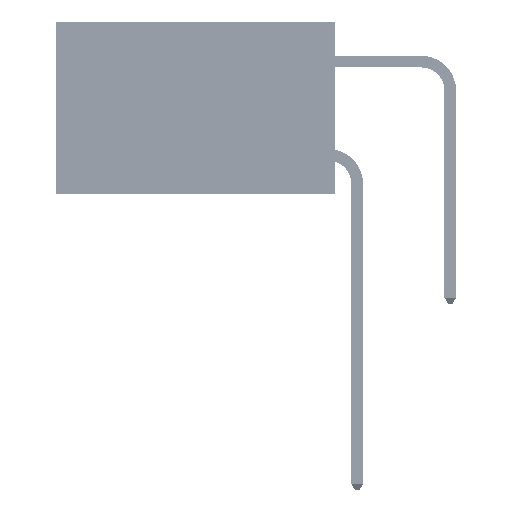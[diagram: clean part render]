
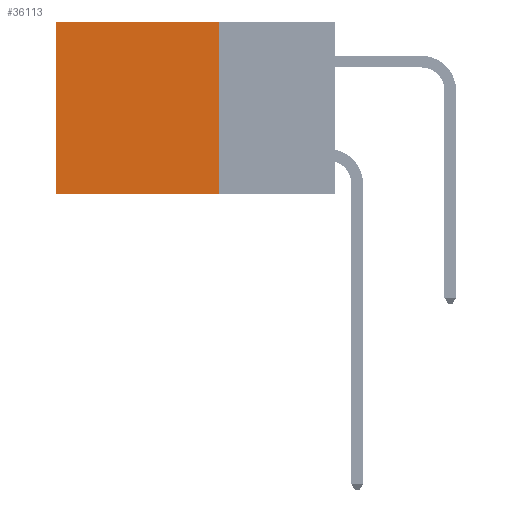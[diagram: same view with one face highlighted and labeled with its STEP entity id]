
A CAD part, left-side view. The second image highlights one B-rep face of the part: STEP entity #36113.
In plain terms, the highlighted planar face has unit normal (-1, 0, 0).
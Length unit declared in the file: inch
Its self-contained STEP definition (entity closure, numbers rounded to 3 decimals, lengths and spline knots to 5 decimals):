
#120 = CARTESIAN_POINT ( 'NONE',  ( 0.2875, 0.25, -0.37 ) ) ;
#1273 = DIRECTION ( 'NONE',  ( 0., 1., 0. ) ) ;
#5257 = EDGE_CURVE ( 'NONE', #51670, #51236, #9615, .T. ) ;
#5672 = DIRECTION ( 'NONE',  ( 1., 0., 0. ) ) ;
#8105 = CARTESIAN_POINT ( 'NONE',  ( 0.2875, 0.25, 0. ) ) ;
#9615 = LINE ( 'NONE', #45702, #12149 ) ;
#9838 = EDGE_LOOP ( 'NONE', ( #26033, #38662, #48596, #29045 ) ) ;
#12149 = VECTOR ( 'NONE', #1273, 39.37008 ) ;
#16026 = EDGE_CURVE ( 'NONE', #17671, #51670, #20615, .T. ) ;
#16264 = EDGE_CURVE ( 'NONE', #17671, #49271, #29444, .T. ) ;
#17465 = VECTOR ( 'NONE', #42611, 39.37008 ) ;
#17671 = VERTEX_POINT ( 'NONE', #19517 ) ;
#19517 = CARTESIAN_POINT ( 'NONE',  ( 0.2875, 0.25, 0. ) ) ;
#20615 = LINE ( 'NONE', #30305, #17465 ) ;
#21214 = CARTESIAN_POINT ( 'NONE',  ( 0.2875, 0.6, -0.37 ) ) ;
#21512 = CARTESIAN_POINT ( 'NONE',  ( 0.2875, 0.25, 0. ) ) ;
#22758 = LINE ( 'NONE', #32452, #39108 ) ;
#25727 = AXIS2_PLACEMENT_3D ( 'NONE', #21512, #5672, #46287 ) ;
#25748 = PLANE ( 'NONE',  #25727 ) ;
#26033 = ORIENTED_EDGE ( 'NONE', *, *, #27079, .T. ) ;
#27079 = EDGE_CURVE ( 'NONE', #49271, #51236, #22758, .T. ) ;
#27839 = DIRECTION ( 'NONE',  ( 0., 1., 0. ) ) ;
#29045 = ORIENTED_EDGE ( 'NONE', *, *, #16264, .T. ) ;
#29444 = LINE ( 'NONE', #8105, #42043 ) ;
#30305 = CARTESIAN_POINT ( 'NONE',  ( 0.2875, 0.25, 0. ) ) ;
#32452 = CARTESIAN_POINT ( 'NONE',  ( 0.2875, 0.6, 0. ) ) ;
#36113 = ADVANCED_FACE ( 'NONE', ( #39462 ), #25748, .F. ) ;
#38662 = ORIENTED_EDGE ( 'NONE', *, *, #5257, .F. ) ;
#39108 = VECTOR ( 'NONE', #48640, 39.37008 ) ;
#39462 = FACE_OUTER_BOUND ( 'NONE', #9838, .T. ) ;
#42043 = VECTOR ( 'NONE', #27839, 39.37008 ) ;
#42611 = DIRECTION ( 'NONE',  ( 0., 0., -1. ) ) ;
#45702 = CARTESIAN_POINT ( 'NONE',  ( 0.2875, 0.25, -0.37 ) ) ;
#45840 = CARTESIAN_POINT ( 'NONE',  ( 0.2875, 0.6, 0. ) ) ;
#46287 = DIRECTION ( 'NONE',  ( 0., 0., -1. ) ) ;
#48596 = ORIENTED_EDGE ( 'NONE', *, *, #16026, .F. ) ;
#48640 = DIRECTION ( 'NONE',  ( 0., 0., -1. ) ) ;
#49271 = VERTEX_POINT ( 'NONE', #45840 ) ;
#51236 = VERTEX_POINT ( 'NONE', #21214 ) ;
#51670 = VERTEX_POINT ( 'NONE', #120 ) ;
